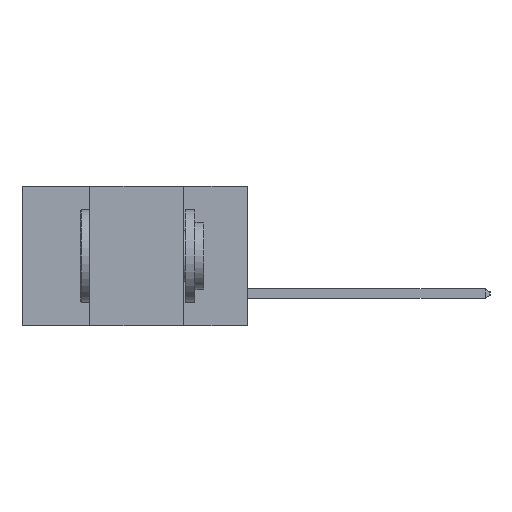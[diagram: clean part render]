
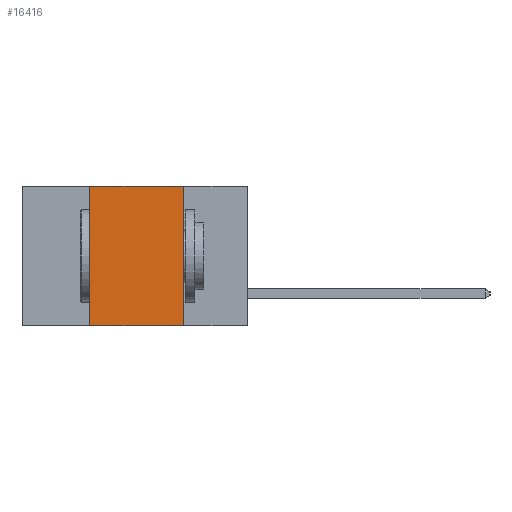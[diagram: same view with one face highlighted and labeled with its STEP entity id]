
A CAD part, left-side view. The second image highlights one B-rep face of the part: STEP entity #16416.
In plain terms, the highlighted planar face has unit normal (-1, 0, 0).
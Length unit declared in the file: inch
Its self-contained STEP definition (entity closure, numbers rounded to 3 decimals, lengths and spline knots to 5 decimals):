
#96 = VECTOR ( 'NONE', #480, 39.37008 ) ;
#480 = DIRECTION ( 'NONE',  ( 0., 0., 1. ) ) ;
#531 = VERTEX_POINT ( 'NONE', #18146 ) ;
#1339 = CARTESIAN_POINT ( 'NONE',  ( 0., 0.6, 0. ) ) ;
#1724 = ORIENTED_EDGE ( 'NONE', *, *, #12289, .F. ) ;
#2281 = DIRECTION ( 'NONE',  ( 0., -1., 0. ) ) ;
#2359 = LINE ( 'NONE', #7685, #12967 ) ;
#2499 = CARTESIAN_POINT ( 'NONE',  ( 0., 0.6, -0.37 ) ) ;
#2607 = EDGE_LOOP ( 'NONE', ( #6024, #1724, #16017, #10067 ) ) ;
#3990 = LINE ( 'NONE', #14847, #96 ) ;
#4099 = AXIS2_PLACEMENT_3D ( 'NONE', #1339, #5727, #15693 ) ;
#4341 = VERTEX_POINT ( 'NONE', #8431 ) ;
#5317 = EDGE_CURVE ( 'NONE', #4341, #8718, #16844, .T. ) ;
#5727 = DIRECTION ( 'NONE',  ( 1., 0., 0. ) ) ;
#6024 = ORIENTED_EDGE ( 'NONE', *, *, #12227, .F. ) ;
#7117 = LINE ( 'NONE', #17269, #10480 ) ;
#7685 = CARTESIAN_POINT ( 'NONE',  ( 0., 0.6, 0. ) ) ;
#8431 = CARTESIAN_POINT ( 'NONE',  ( 0., 0.42, -0.37 ) ) ;
#8718 = VERTEX_POINT ( 'NONE', #11082 ) ;
#10067 = ORIENTED_EDGE ( 'NONE', *, *, #5317, .T. ) ;
#10480 = VECTOR ( 'NONE', #11838, 39.37008 ) ;
#11082 = CARTESIAN_POINT ( 'NONE',  ( 0., 0.17, -0.37 ) ) ;
#11838 = DIRECTION ( 'NONE',  ( 0., 0., -1. ) ) ;
#12227 = EDGE_CURVE ( 'NONE', #531, #8718, #7117, .T. ) ;
#12289 = EDGE_CURVE ( 'NONE', #12498, #531, #2359, .T. ) ;
#12498 = VERTEX_POINT ( 'NONE', #13898 ) ;
#12967 = VECTOR ( 'NONE', #16145, 39.37008 ) ;
#13898 = CARTESIAN_POINT ( 'NONE',  ( 0., 0.42, 0. ) ) ;
#14154 = VECTOR ( 'NONE', #2281, 39.37008 ) ;
#14325 = PLANE ( 'NONE',  #4099 ) ;
#14847 = CARTESIAN_POINT ( 'NONE',  ( 0., 0.42, -0.37 ) ) ;
#15514 = EDGE_CURVE ( 'NONE', #4341, #12498, #3990, .T. ) ;
#15693 = DIRECTION ( 'NONE',  ( 0., 0., -1. ) ) ;
#16017 = ORIENTED_EDGE ( 'NONE', *, *, #15514, .F. ) ;
#16145 = DIRECTION ( 'NONE',  ( 0., -1., 0. ) ) ;
#16416 = ADVANCED_FACE ( 'NONE', ( #17152 ), #14325, .F. ) ;
#16844 = LINE ( 'NONE', #2499, #14154 ) ;
#17152 = FACE_OUTER_BOUND ( 'NONE', #2607, .T. ) ;
#17269 = CARTESIAN_POINT ( 'NONE',  ( 0., 0.17, -0.37 ) ) ;
#18146 = CARTESIAN_POINT ( 'NONE',  ( 0., 0.17, 0. ) ) ;
